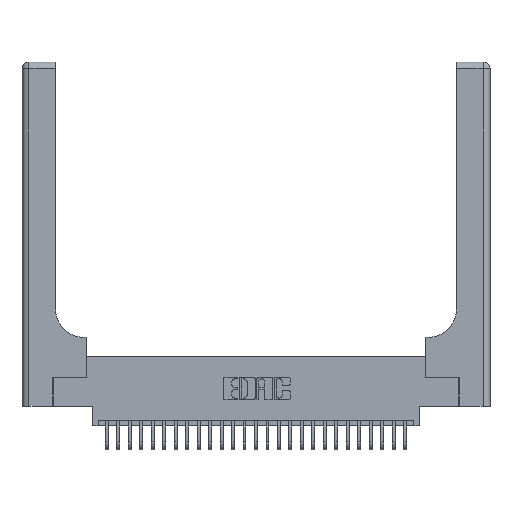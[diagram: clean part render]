
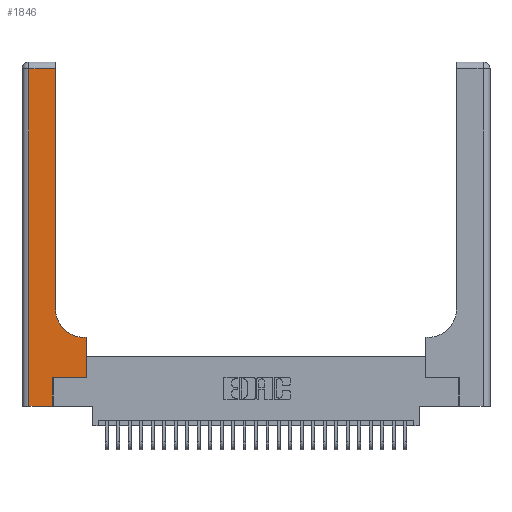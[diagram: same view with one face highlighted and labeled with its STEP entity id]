
A CAD part, top view. The second image highlights one B-rep face of the part: STEP entity #1846.
In plain terms, the highlighted planar face has unit normal (0, 0, 1).
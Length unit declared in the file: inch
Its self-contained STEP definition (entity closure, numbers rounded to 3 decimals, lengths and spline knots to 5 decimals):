
#10 = LINE ( 'NONE', #6139, #23400 ) ;
#243 = DIRECTION ( 'NONE',  ( -1., 0., 0. ) ) ;
#945 = LINE ( 'NONE', #9568, #11233 ) ;
#981 = EDGE_CURVE ( 'NONE', #22839, #7726, #10, .T. ) ;
#1465 = ORIENTED_EDGE ( 'NONE', *, *, #22868, .T. ) ;
#1729 = VERTEX_POINT ( 'NONE', #20767 ) ;
#1846 = ADVANCED_FACE ( 'NONE', ( #21880 ), #4924, .F. ) ;
#1990 = EDGE_CURVE ( 'NONE', #19719, #6417, #12073, .T. ) ;
#4068 = DIRECTION ( 'NONE',  ( -1., 0., 0. ) ) ;
#4277 = CARTESIAN_POINT ( 'NONE',  ( 0., 0., 0.37 ) ) ;
#4924 = PLANE ( 'NONE',  #10703 ) ;
#5145 = CARTESIAN_POINT ( 'NONE',  ( 0.269, 0.25, 0.37 ) ) ;
#5592 = LINE ( 'NONE', #15666, #19389 ) ;
#5873 = DIRECTION ( 'NONE',  ( 0., 1., 0. ) ) ;
#6060 = DIRECTION ( 'NONE',  ( 0., 1., 0. ) ) ;
#6139 = CARTESIAN_POINT ( 'NONE',  ( 0.2915, 3., 0.37 ) ) ;
#6417 = VERTEX_POINT ( 'NONE', #7754 ) ;
#7726 = VERTEX_POINT ( 'NONE', #21440 ) ;
#7754 = CARTESIAN_POINT ( 'NONE',  ( 0.5585, 0.25, 0.37 ) ) ;
#9189 = ORIENTED_EDGE ( 'NONE', *, *, #15244, .T. ) ;
#9568 = CARTESIAN_POINT ( 'NONE',  ( 0.06, 3., 0.37 ) ) ;
#10703 = AXIS2_PLACEMENT_3D ( 'NONE', #25865, #14295, #243 ) ;
#11233 = VECTOR ( 'NONE', #18900, 39.37008 ) ;
#11546 = VECTOR ( 'NONE', #16327, 39.37008 ) ;
#12073 = LINE ( 'NONE', #24432, #29840 ) ;
#12118 = CARTESIAN_POINT ( 'NONE',  ( 0.5415, 0.85, 0.37 ) ) ;
#12380 = EDGE_CURVE ( 'NONE', #7726, #24792, #17686, .T. ) ;
#12470 = ORIENTED_EDGE ( 'NONE', *, *, #12380, .T. ) ;
#13150 = LINE ( 'NONE', #4277, #18570 ) ;
#13935 = ORIENTED_EDGE ( 'NONE', *, *, #25349, .T. ) ;
#14229 = CARTESIAN_POINT ( 'NONE',  ( 0.06, 2.94, 0.37 ) ) ;
#14295 = DIRECTION ( 'NONE',  ( 0., 0., -1. ) ) ;
#14459 = DIRECTION ( 'NONE',  ( 1., 0., 0. ) ) ;
#15244 = EDGE_CURVE ( 'NONE', #17624, #26532, #5592, .T. ) ;
#15465 = EDGE_CURVE ( 'NONE', #26532, #22839, #18290, .T. ) ;
#15666 = CARTESIAN_POINT ( 'NONE',  ( 0.2915, 0.6, 0.37 ) ) ;
#16327 = DIRECTION ( 'NONE',  ( -1., 0., 0. ) ) ;
#17165 = ORIENTED_EDGE ( 'NONE', *, *, #981, .T. ) ;
#17624 = VERTEX_POINT ( 'NONE', #21827 ) ;
#17686 = LINE ( 'NONE', #18540, #11546 ) ;
#18290 = CIRCLE ( 'NONE', #22387, 0.25 ) ;
#18540 = CARTESIAN_POINT ( 'NONE',  ( 0., 2.94, 0.37 ) ) ;
#18570 = VECTOR ( 'NONE', #22877, 39.37008 ) ;
#18616 = CARTESIAN_POINT ( 'NONE',  ( 0.269, 0., 0.37 ) ) ;
#18900 = DIRECTION ( 'NONE',  ( 0., -1., 0. ) ) ;
#19389 = VECTOR ( 'NONE', #4068, 39.37008 ) ;
#19719 = VERTEX_POINT ( 'NONE', #5145 ) ;
#20059 = CARTESIAN_POINT ( 'NONE',  ( 0.06, 0., 0.37 ) ) ;
#20374 = LINE ( 'NONE', #22144, #25863 ) ;
#20767 = CARTESIAN_POINT ( 'NONE',  ( 0.269, 0., 0.37 ) ) ;
#20809 = ORIENTED_EDGE ( 'NONE', *, *, #1990, .T. ) ;
#20971 = DIRECTION ( 'NONE',  ( 0., 1., 0. ) ) ;
#21440 = CARTESIAN_POINT ( 'NONE',  ( 0.2915, 2.94, 0.37 ) ) ;
#21805 = VECTOR ( 'NONE', #20971, 39.37008 ) ;
#21827 = CARTESIAN_POINT ( 'NONE',  ( 0.5585, 0.6, 0.37 ) ) ;
#21880 = FACE_OUTER_BOUND ( 'NONE', #23732, .T. ) ;
#22144 = CARTESIAN_POINT ( 'NONE',  ( 0.5585, 0.25, 0.37 ) ) ;
#22387 = AXIS2_PLACEMENT_3D ( 'NONE', #12118, #28383, #14459 ) ;
#22839 = VERTEX_POINT ( 'NONE', #29661 ) ;
#22868 = EDGE_CURVE ( 'NONE', #27161, #1729, #13150, .T. ) ;
#22877 = DIRECTION ( 'NONE',  ( 1., 0., 0. ) ) ;
#23400 = VECTOR ( 'NONE', #6060, 39.37008 ) ;
#23732 = EDGE_LOOP ( 'NONE', ( #17165, #12470, #25560, #1465, #13935, #20809, #27015, #9189, #28484 ) ) ;
#24337 = DIRECTION ( 'NONE',  ( 1., 0., 0. ) ) ;
#24432 = CARTESIAN_POINT ( 'NONE',  ( 0.269, 0.25, 0.37 ) ) ;
#24487 = EDGE_CURVE ( 'NONE', #6417, #17624, #20374, .T. ) ;
#24792 = VERTEX_POINT ( 'NONE', #14229 ) ;
#25349 = EDGE_CURVE ( 'NONE', #1729, #19719, #28023, .T. ) ;
#25560 = ORIENTED_EDGE ( 'NONE', *, *, #25992, .T. ) ;
#25863 = VECTOR ( 'NONE', #5873, 39.37008 ) ;
#25865 = CARTESIAN_POINT ( 'NONE',  ( 0., 3., 0.37 ) ) ;
#25992 = EDGE_CURVE ( 'NONE', #24792, #27161, #945, .T. ) ;
#26532 = VERTEX_POINT ( 'NONE', #27758 ) ;
#27015 = ORIENTED_EDGE ( 'NONE', *, *, #24487, .T. ) ;
#27161 = VERTEX_POINT ( 'NONE', #20059 ) ;
#27758 = CARTESIAN_POINT ( 'NONE',  ( 0.5415, 0.6, 0.37 ) ) ;
#28023 = LINE ( 'NONE', #18616, #21805 ) ;
#28383 = DIRECTION ( 'NONE',  ( 0., 0., -1. ) ) ;
#28484 = ORIENTED_EDGE ( 'NONE', *, *, #15465, .T. ) ;
#29661 = CARTESIAN_POINT ( 'NONE',  ( 0.2915, 0.85, 0.37 ) ) ;
#29840 = VECTOR ( 'NONE', #24337, 39.37008 ) ;
